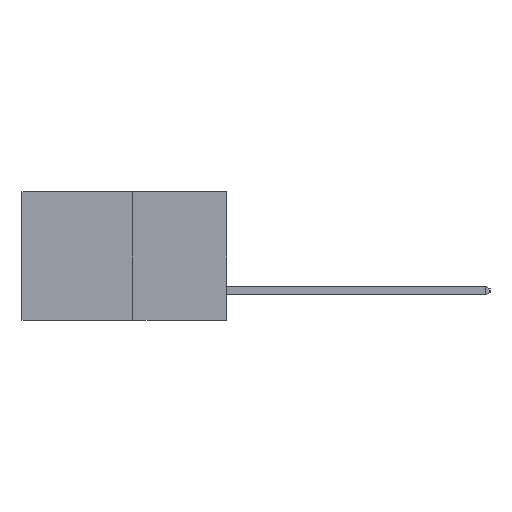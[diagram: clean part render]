
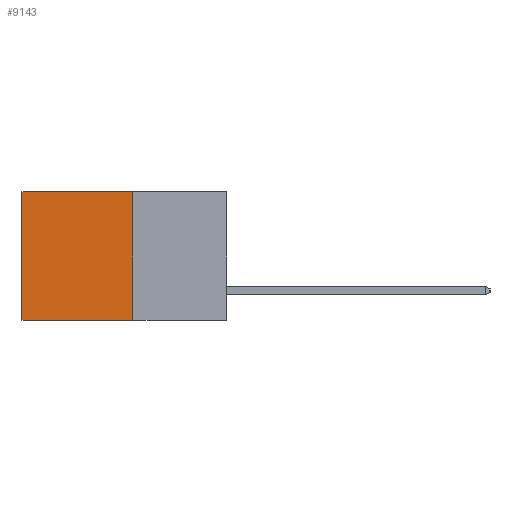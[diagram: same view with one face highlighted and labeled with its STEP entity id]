
A CAD part, left-side view. The second image highlights one B-rep face of the part: STEP entity #9143.
In plain terms, the highlighted planar face has unit normal (-1, 0, 0).
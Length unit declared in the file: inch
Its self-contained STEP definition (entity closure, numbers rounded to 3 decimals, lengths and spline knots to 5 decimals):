
#777 = LINE ( 'NONE', #9415, #4896 ) ;
#1049 = VECTOR ( 'NONE', #4115, 39.37008 ) ;
#1243 = ORIENTED_EDGE ( 'NONE', *, *, #5573, .T. ) ;
#1255 = DIRECTION ( 'NONE',  ( 0., 0., -1. ) ) ;
#1403 = FACE_OUTER_BOUND ( 'NONE', #6359, .T. ) ;
#1454 = CARTESIAN_POINT ( 'NONE',  ( 0.277, 0.27, -0.37 ) ) ;
#2213 = VECTOR ( 'NONE', #4132, 39.37008 ) ;
#2525 = CARTESIAN_POINT ( 'NONE',  ( 0.277, 0.27, 0. ) ) ;
#3163 = VERTEX_POINT ( 'NONE', #8464 ) ;
#3195 = AXIS2_PLACEMENT_3D ( 'NONE', #4331, #5907, #1255 ) ;
#4115 = DIRECTION ( 'NONE',  ( 0., 1., 0. ) ) ;
#4132 = DIRECTION ( 'NONE',  ( 0., 1., 0. ) ) ;
#4331 = CARTESIAN_POINT ( 'NONE',  ( 0.277, 0.27, -0.37 ) ) ;
#4554 = VERTEX_POINT ( 'NONE', #7543 ) ;
#4896 = VECTOR ( 'NONE', #7894, 39.37008 ) ;
#5187 = VECTOR ( 'NONE', #5715, 39.37008 ) ;
#5441 = LINE ( 'NONE', #9470, #5187 ) ;
#5573 = EDGE_CURVE ( 'NONE', #4554, #3163, #6914, .T. ) ;
#5715 = DIRECTION ( 'NONE',  ( 0., 0., -1. ) ) ;
#5839 = VERTEX_POINT ( 'NONE', #8137 ) ;
#5907 = DIRECTION ( 'NONE',  ( 1., 0., 0. ) ) ;
#6248 = EDGE_CURVE ( 'NONE', #8376, #5839, #6331, .T. ) ;
#6331 = LINE ( 'NONE', #6408, #2213 ) ;
#6359 = EDGE_LOOP ( 'NONE', ( #8124, #8447, #7652, #1243 ) ) ;
#6408 = CARTESIAN_POINT ( 'NONE',  ( 0.277, 0.27, -0.37 ) ) ;
#6834 = EDGE_CURVE ( 'NONE', #3163, #5839, #777, .T. ) ;
#6914 = LINE ( 'NONE', #2525, #1049 ) ;
#7543 = CARTESIAN_POINT ( 'NONE',  ( 0.277, 0.27, 0. ) ) ;
#7652 = ORIENTED_EDGE ( 'NONE', *, *, #8442, .F. ) ;
#7894 = DIRECTION ( 'NONE',  ( 0., 0., -1. ) ) ;
#8093 = PLANE ( 'NONE',  #3195 ) ;
#8124 = ORIENTED_EDGE ( 'NONE', *, *, #6834, .T. ) ;
#8137 = CARTESIAN_POINT ( 'NONE',  ( 0.277, 0.59, -0.37 ) ) ;
#8376 = VERTEX_POINT ( 'NONE', #1454 ) ;
#8442 = EDGE_CURVE ( 'NONE', #4554, #8376, #5441, .T. ) ;
#8447 = ORIENTED_EDGE ( 'NONE', *, *, #6248, .F. ) ;
#8464 = CARTESIAN_POINT ( 'NONE',  ( 0.277, 0.59, 0. ) ) ;
#9143 = ADVANCED_FACE ( 'NONE', ( #1403 ), #8093, .F. ) ;
#9415 = CARTESIAN_POINT ( 'NONE',  ( 0.277, 0.59, -0.37 ) ) ;
#9470 = CARTESIAN_POINT ( 'NONE',  ( 0.277, 0.27, -0.37 ) ) ;
